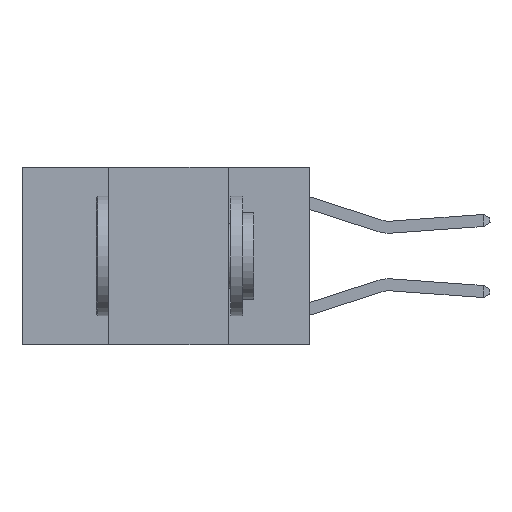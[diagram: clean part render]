
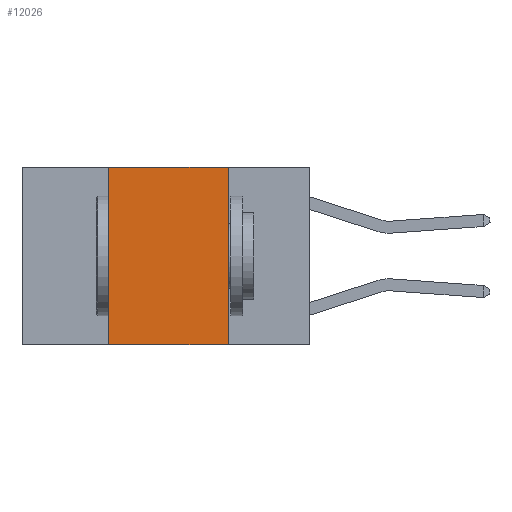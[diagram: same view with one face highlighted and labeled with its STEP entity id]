
A CAD part, left-side view. The second image highlights one B-rep face of the part: STEP entity #12026.
In plain terms, the highlighted planar face has unit normal (-1, 0, 0).
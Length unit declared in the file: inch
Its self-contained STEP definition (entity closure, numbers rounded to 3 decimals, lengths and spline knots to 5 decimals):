
#289 = FACE_OUTER_BOUND ( 'NONE', #2358, .T. ) ;
#761 = ORIENTED_EDGE ( 'NONE', *, *, #4673, .F. ) ;
#1373 = DIRECTION ( 'NONE',  ( 1., 0., 0. ) ) ;
#2308 = VERTEX_POINT ( 'NONE', #9802 ) ;
#2358 = EDGE_LOOP ( 'NONE', ( #12023, #761, #2504, #12028 ) ) ;
#2504 = ORIENTED_EDGE ( 'NONE', *, *, #7504, .F. ) ;
#3610 = CARTESIAN_POINT ( 'NONE',  ( 0., 0.17, 0. ) ) ;
#4546 = DIRECTION ( 'NONE',  ( 0., 0., -1. ) ) ;
#4611 = CARTESIAN_POINT ( 'NONE',  ( 0., 0.42, 0. ) ) ;
#4673 = EDGE_CURVE ( 'NONE', #9136, #12066, #8011, .T. ) ;
#5000 = AXIS2_PLACEMENT_3D ( 'NONE', #12301, #1373, #4546 ) ;
#5420 = DIRECTION ( 'NONE',  ( 0., 0., -1. ) ) ;
#5626 = DIRECTION ( 'NONE',  ( 0., 0., 1. ) ) ;
#6072 = VECTOR ( 'NONE', #5420, 39.37008 ) ;
#6982 = VECTOR ( 'NONE', #5626, 39.37008 ) ;
#7329 = DIRECTION ( 'NONE',  ( 0., -1., 0. ) ) ;
#7335 = EDGE_CURVE ( 'NONE', #12066, #2308, #9555, .T. ) ;
#7504 = EDGE_CURVE ( 'NONE', #13402, #9136, #12211, .T. ) ;
#7864 = DIRECTION ( 'NONE',  ( 0., -1., 0. ) ) ;
#8011 = LINE ( 'NONE', #12371, #9873 ) ;
#8304 = EDGE_CURVE ( 'NONE', #13402, #2308, #10530, .T. ) ;
#8506 = CARTESIAN_POINT ( 'NONE',  ( 0., 0.17, 0. ) ) ;
#8911 = CARTESIAN_POINT ( 'NONE',  ( 0., 0.42, 0. ) ) ;
#9136 = VERTEX_POINT ( 'NONE', #8911 ) ;
#9555 = LINE ( 'NONE', #8506, #6072 ) ;
#9802 = CARTESIAN_POINT ( 'NONE',  ( 0., 0.17, -0.37 ) ) ;
#9873 = VECTOR ( 'NONE', #7864, 39.37008 ) ;
#10530 = LINE ( 'NONE', #12770, #13653 ) ;
#12023 = ORIENTED_EDGE ( 'NONE', *, *, #7335, .F. ) ;
#12026 = ADVANCED_FACE ( 'NONE', ( #289 ), #13531, .F. ) ;
#12028 = ORIENTED_EDGE ( 'NONE', *, *, #8304, .T. ) ;
#12066 = VERTEX_POINT ( 'NONE', #3610 ) ;
#12211 = LINE ( 'NONE', #4611, #6982 ) ;
#12301 = CARTESIAN_POINT ( 'NONE',  ( 0., 0.6, 0. ) ) ;
#12371 = CARTESIAN_POINT ( 'NONE',  ( 0., 0.6, 0. ) ) ;
#12375 = CARTESIAN_POINT ( 'NONE',  ( 0., 0.42, -0.37 ) ) ;
#12770 = CARTESIAN_POINT ( 'NONE',  ( 0., 0.6, -0.37 ) ) ;
#13402 = VERTEX_POINT ( 'NONE', #12375 ) ;
#13531 = PLANE ( 'NONE',  #5000 ) ;
#13653 = VECTOR ( 'NONE', #7329, 39.37008 ) ;
